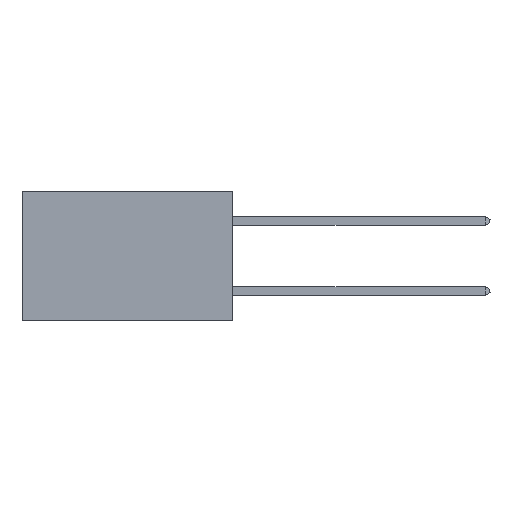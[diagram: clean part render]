
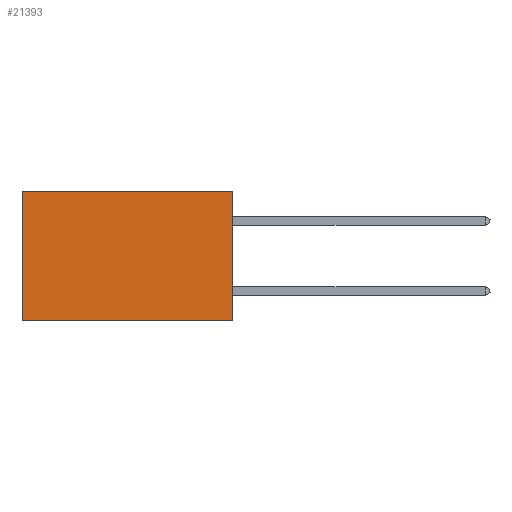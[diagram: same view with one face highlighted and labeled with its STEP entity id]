
A CAD part, left-side view. The second image highlights one B-rep face of the part: STEP entity #21393.
In plain terms, the highlighted planar face has unit normal (-1, 0, 0).
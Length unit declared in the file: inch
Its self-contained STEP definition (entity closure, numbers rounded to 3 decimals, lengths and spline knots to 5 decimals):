
#2942 = DIRECTION ( 'NONE',  ( 0., 0., -1. ) ) ;
#3254 = VECTOR ( 'NONE', #18847, 39.37008 ) ;
#3358 = VERTEX_POINT ( 'NONE', #37688 ) ;
#3807 = ORIENTED_EDGE ( 'NONE', *, *, #10931, .T. ) ;
#4227 = ORIENTED_EDGE ( 'NONE', *, *, #14588, .T. ) ;
#5394 = DIRECTION ( 'NONE',  ( 0., 0., -1. ) ) ;
#6088 = LINE ( 'NONE', #34609, #36222 ) ;
#7620 = LINE ( 'NONE', #14933, #32684 ) ;
#7939 = EDGE_LOOP ( 'NONE', ( #4227, #15697, #35698, #3807 ) ) ;
#10931 = EDGE_CURVE ( 'NONE', #31478, #36781, #35647, .T. ) ;
#11893 = DIRECTION ( 'NONE',  ( 0., 1., 0. ) ) ;
#12172 = DIRECTION ( 'NONE',  ( 0., 0., -1. ) ) ;
#12915 = CARTESIAN_POINT ( 'NONE',  ( 0.2875, 0., 0. ) ) ;
#13023 = CARTESIAN_POINT ( 'NONE',  ( 0.2875, 0., 0. ) ) ;
#13545 = LINE ( 'NONE', #20383, #20323 ) ;
#13820 = FACE_OUTER_BOUND ( 'NONE', #7939, .T. ) ;
#14588 = EDGE_CURVE ( 'NONE', #36781, #24345, #6088, .T. ) ;
#14933 = CARTESIAN_POINT ( 'NONE',  ( 0.2875, 0., -0.37 ) ) ;
#15697 = ORIENTED_EDGE ( 'NONE', *, *, #18895, .F. ) ;
#18847 = DIRECTION ( 'NONE',  ( 0., 1., 0. ) ) ;
#18895 = EDGE_CURVE ( 'NONE', #3358, #24345, #7620, .T. ) ;
#19398 = EDGE_CURVE ( 'NONE', #31478, #3358, #13545, .T. ) ;
#20323 = VECTOR ( 'NONE', #2942, 39.37008 ) ;
#20383 = CARTESIAN_POINT ( 'NONE',  ( 0.2875, 0., 0. ) ) ;
#21048 = CARTESIAN_POINT ( 'NONE',  ( 0.2875, 0., 0. ) ) ;
#21393 = ADVANCED_FACE ( 'NONE', ( #13820 ), #35319, .F. ) ;
#24345 = VERTEX_POINT ( 'NONE', #36966 ) ;
#28035 = CARTESIAN_POINT ( 'NONE',  ( 0.2875, 0.6, 0. ) ) ;
#29964 = DIRECTION ( 'NONE',  ( 1., 0., 0. ) ) ;
#30050 = AXIS2_PLACEMENT_3D ( 'NONE', #21048, #29964, #12172 ) ;
#31478 = VERTEX_POINT ( 'NONE', #13023 ) ;
#32684 = VECTOR ( 'NONE', #11893, 39.37008 ) ;
#34609 = CARTESIAN_POINT ( 'NONE',  ( 0.2875, 0.6, 0. ) ) ;
#35319 = PLANE ( 'NONE',  #30050 ) ;
#35647 = LINE ( 'NONE', #12915, #3254 ) ;
#35698 = ORIENTED_EDGE ( 'NONE', *, *, #19398, .F. ) ;
#36222 = VECTOR ( 'NONE', #5394, 39.37008 ) ;
#36781 = VERTEX_POINT ( 'NONE', #28035 ) ;
#36966 = CARTESIAN_POINT ( 'NONE',  ( 0.2875, 0.6, -0.37 ) ) ;
#37688 = CARTESIAN_POINT ( 'NONE',  ( 0.2875, 0., -0.37 ) ) ;
